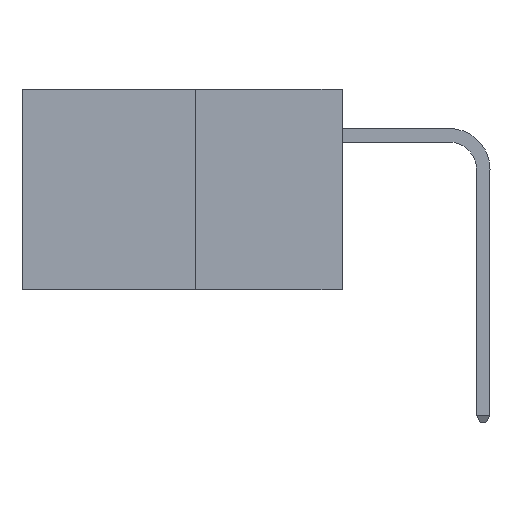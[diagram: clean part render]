
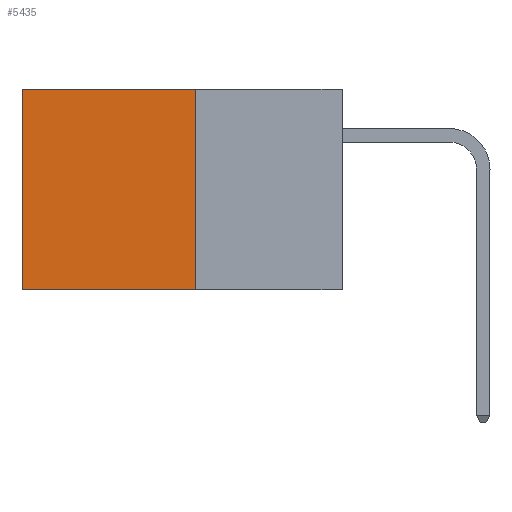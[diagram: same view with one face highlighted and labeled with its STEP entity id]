
A CAD part, left-side view. The second image highlights one B-rep face of the part: STEP entity #5435.
In plain terms, the highlighted planar face has unit normal (-1, 0, 0).
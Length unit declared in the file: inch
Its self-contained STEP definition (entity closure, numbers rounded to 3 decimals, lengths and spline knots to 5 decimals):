
#707 = VECTOR ( 'NONE', #5327, 39.37008 ) ;
#786 = VERTEX_POINT ( 'NONE', #6618 ) ;
#1002 = CARTESIAN_POINT ( 'NONE',  ( 0.277, 0.27, 0. ) ) ;
#1038 = DIRECTION ( 'NONE',  ( 0., 0., -1. ) ) ;
#1067 = DIRECTION ( 'NONE',  ( 1., 0., 0. ) ) ;
#1159 = CARTESIAN_POINT ( 'NONE',  ( 0.277, 0.27, -0.37 ) ) ;
#1197 = PLANE ( 'NONE',  #6729 ) ;
#1389 = EDGE_CURVE ( 'NONE', #6708, #8162, #9445, .T. ) ;
#1429 = LINE ( 'NONE', #3868, #6198 ) ;
#1751 = CARTESIAN_POINT ( 'NONE',  ( 0.277, 0.59, -0.37 ) ) ;
#2701 = CARTESIAN_POINT ( 'NONE',  ( 0.277, 0.27, -0.37 ) ) ;
#3202 = EDGE_CURVE ( 'NONE', #9766, #6708, #1429, .T. ) ;
#3868 = CARTESIAN_POINT ( 'NONE',  ( 0.277, 0.27, -0.37 ) ) ;
#3908 = CARTESIAN_POINT ( 'NONE',  ( 0.277, 0.59, -0.37 ) ) ;
#4513 = DIRECTION ( 'NONE',  ( 0., 1., 0. ) ) ;
#4586 = ORIENTED_EDGE ( 'NONE', *, *, #5850, .T. ) ;
#5217 = EDGE_CURVE ( 'NONE', #786, #8162, #9512, .T. ) ;
#5292 = DIRECTION ( 'NONE',  ( 0., 0., -1. ) ) ;
#5327 = DIRECTION ( 'NONE',  ( 0., 1., 0. ) ) ;
#5435 = ADVANCED_FACE ( 'NONE', ( #7432 ), #1197, .F. ) ;
#5850 = EDGE_CURVE ( 'NONE', #9766, #786, #10078, .T. ) ;
#5959 = CARTESIAN_POINT ( 'NONE',  ( 0.277, 0.27, 0. ) ) ;
#6198 = VECTOR ( 'NONE', #5292, 39.37008 ) ;
#6277 = DIRECTION ( 'NONE',  ( 0., 0., -1. ) ) ;
#6618 = CARTESIAN_POINT ( 'NONE',  ( 0.277, 0.59, 0. ) ) ;
#6708 = VERTEX_POINT ( 'NONE', #2701 ) ;
#6729 = AXIS2_PLACEMENT_3D ( 'NONE', #1159, #1067, #1038 ) ;
#7432 = FACE_OUTER_BOUND ( 'NONE', #9625, .T. ) ;
#7864 = VECTOR ( 'NONE', #6277, 39.37008 ) ;
#8006 = CARTESIAN_POINT ( 'NONE',  ( 0.277, 0.27, -0.37 ) ) ;
#8162 = VERTEX_POINT ( 'NONE', #3908 ) ;
#8420 = VECTOR ( 'NONE', #4513, 39.37008 ) ;
#8589 = ORIENTED_EDGE ( 'NONE', *, *, #3202, .F. ) ;
#8783 = ORIENTED_EDGE ( 'NONE', *, *, #1389, .F. ) ;
#9224 = ORIENTED_EDGE ( 'NONE', *, *, #5217, .T. ) ;
#9445 = LINE ( 'NONE', #8006, #707 ) ;
#9512 = LINE ( 'NONE', #1751, #7864 ) ;
#9625 = EDGE_LOOP ( 'NONE', ( #9224, #8783, #8589, #4586 ) ) ;
#9766 = VERTEX_POINT ( 'NONE', #1002 ) ;
#10078 = LINE ( 'NONE', #5959, #8420 ) ;
